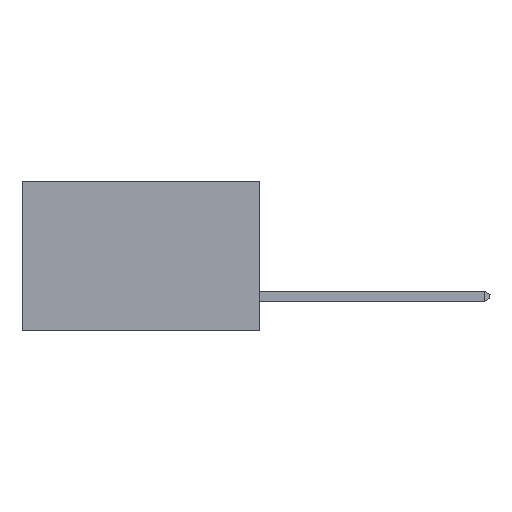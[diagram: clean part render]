
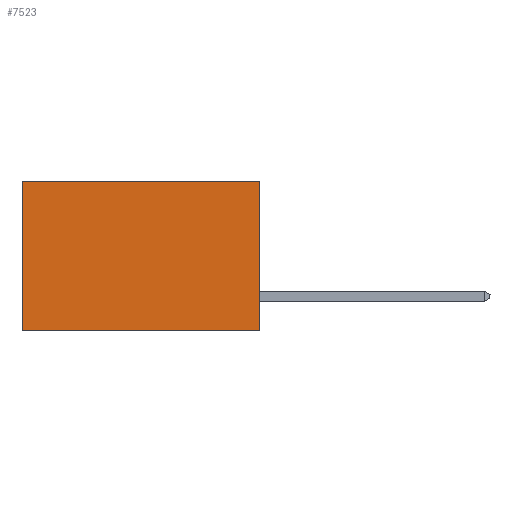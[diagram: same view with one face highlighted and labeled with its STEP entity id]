
A CAD part, left-side view. The second image highlights one B-rep face of the part: STEP entity #7523.
In plain terms, the highlighted planar face has unit normal (-1, 0, 0).
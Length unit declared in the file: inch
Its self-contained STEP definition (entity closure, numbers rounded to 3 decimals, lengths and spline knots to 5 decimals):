
#462 = VECTOR ( 'NONE', #3223, 39.37008 ) ;
#713 = VECTOR ( 'NONE', #5634, 39.37008 ) ;
#1244 = EDGE_CURVE ( 'NONE', #7369, #10694, #11582, .T. ) ;
#1303 = EDGE_CURVE ( 'NONE', #12539, #5524, #5928, .T. ) ;
#1337 = CARTESIAN_POINT ( 'NONE',  ( 0.277, 0.59, -0.37 ) ) ;
#1549 = ORIENTED_EDGE ( 'NONE', *, *, #1303, .T. ) ;
#3223 = DIRECTION ( 'NONE',  ( 0., 1., 0. ) ) ;
#3664 = ORIENTED_EDGE ( 'NONE', *, *, #8577, .T. ) ;
#4769 = CARTESIAN_POINT ( 'NONE',  ( 0.277, 0.59, 0. ) ) ;
#4790 = CARTESIAN_POINT ( 'NONE',  ( 0.277, 0., 0. ) ) ;
#5377 = VECTOR ( 'NONE', #7301, 39.37008 ) ;
#5414 = CARTESIAN_POINT ( 'NONE',  ( 0.277, 0.59, -0.37 ) ) ;
#5524 = VERTEX_POINT ( 'NONE', #1337 ) ;
#5634 = DIRECTION ( 'NONE',  ( 0., 0., -1. ) ) ;
#5684 = EDGE_CURVE ( 'NONE', #10694, #5524, #8373, .T. ) ;
#5928 = LINE ( 'NONE', #5414, #8865 ) ;
#6299 = EDGE_LOOP ( 'NONE', ( #1549, #9915, #13235, #3664 ) ) ;
#7301 = DIRECTION ( 'NONE',  ( 0., 1., 0. ) ) ;
#7369 = VERTEX_POINT ( 'NONE', #4790 ) ;
#7523 = ADVANCED_FACE ( 'NONE', ( #8971 ), #13422, .F. ) ;
#7524 = AXIS2_PLACEMENT_3D ( 'NONE', #12505, #12842, #12571 ) ;
#7618 = CARTESIAN_POINT ( 'NONE',  ( 0.277, 0., -0.37 ) ) ;
#8373 = LINE ( 'NONE', #7618, #5377 ) ;
#8403 = CARTESIAN_POINT ( 'NONE',  ( 0.277, 0., 0. ) ) ;
#8533 = CARTESIAN_POINT ( 'NONE',  ( 0.277, 0., -0.37 ) ) ;
#8577 = EDGE_CURVE ( 'NONE', #7369, #12539, #11376, .T. ) ;
#8865 = VECTOR ( 'NONE', #10557, 39.37008 ) ;
#8971 = FACE_OUTER_BOUND ( 'NONE', #6299, .T. ) ;
#9915 = ORIENTED_EDGE ( 'NONE', *, *, #5684, .F. ) ;
#10557 = DIRECTION ( 'NONE',  ( 0., 0., -1. ) ) ;
#10628 = CARTESIAN_POINT ( 'NONE',  ( 0.277, 0., -0.37 ) ) ;
#10694 = VERTEX_POINT ( 'NONE', #8533 ) ;
#11376 = LINE ( 'NONE', #8403, #462 ) ;
#11582 = LINE ( 'NONE', #10628, #713 ) ;
#12505 = CARTESIAN_POINT ( 'NONE',  ( 0.277, 0., -0.37 ) ) ;
#12539 = VERTEX_POINT ( 'NONE', #4769 ) ;
#12571 = DIRECTION ( 'NONE',  ( 0., 0., -1. ) ) ;
#12842 = DIRECTION ( 'NONE',  ( 1., 0., 0. ) ) ;
#13235 = ORIENTED_EDGE ( 'NONE', *, *, #1244, .F. ) ;
#13422 = PLANE ( 'NONE',  #7524 ) ;
